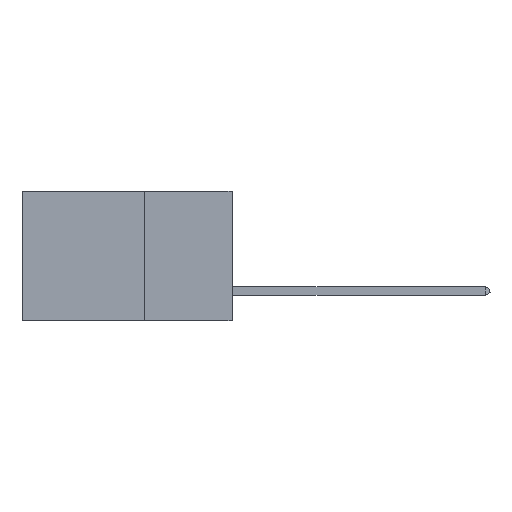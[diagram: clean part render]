
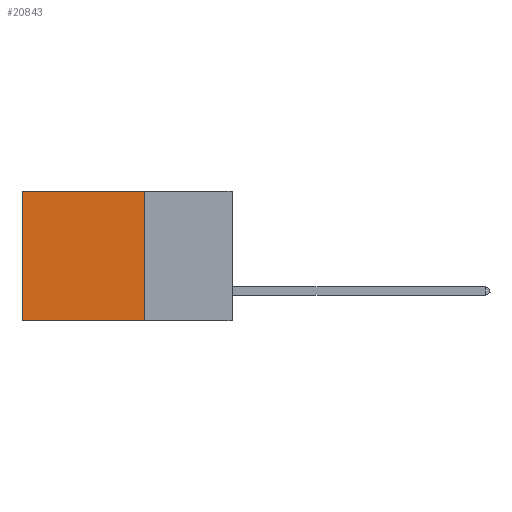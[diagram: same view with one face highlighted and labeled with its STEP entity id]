
A CAD part, left-side view. The second image highlights one B-rep face of the part: STEP entity #20843.
In plain terms, the highlighted planar face has unit normal (-1, 0, 0).
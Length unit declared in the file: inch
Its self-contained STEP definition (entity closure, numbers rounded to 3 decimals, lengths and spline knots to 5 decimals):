
#1390 = LINE ( 'NONE', #25113, #13001 ) ;
#1434 = EDGE_CURVE ( 'NONE', #14051, #10631, #1390, .T. ) ;
#2097 = DIRECTION ( 'NONE',  ( 0., 0., -1. ) ) ;
#3875 = LINE ( 'NONE', #4711, #16712 ) ;
#4231 = DIRECTION ( 'NONE',  ( 0., 1., 0. ) ) ;
#4318 = CARTESIAN_POINT ( 'NONE',  ( 0.2875, 0.25, -0.37 ) ) ;
#4711 = CARTESIAN_POINT ( 'NONE',  ( 0.2875, 0.25, 0. ) ) ;
#4756 = CARTESIAN_POINT ( 'NONE',  ( 0.2875, 0.6, 0. ) ) ;
#4985 = LINE ( 'NONE', #17967, #7149 ) ;
#5354 = LINE ( 'NONE', #4318, #6259 ) ;
#5360 = CARTESIAN_POINT ( 'NONE',  ( 0.2875, 0.6, -0.37 ) ) ;
#5842 = FACE_OUTER_BOUND ( 'NONE', #7116, .T. ) ;
#6259 = VECTOR ( 'NONE', #4231, 39.37008 ) ;
#7116 = EDGE_LOOP ( 'NONE', ( #17181, #24095, #25211, #17843 ) ) ;
#7149 = VECTOR ( 'NONE', #22436, 39.37008 ) ;
#8126 = DIRECTION ( 'NONE',  ( 1., 0., 0. ) ) ;
#10112 = EDGE_CURVE ( 'NONE', #25941, #14051, #3875, .T. ) ;
#10631 = VERTEX_POINT ( 'NONE', #5360 ) ;
#11457 = CARTESIAN_POINT ( 'NONE',  ( 0.2875, 0.25, -0.37 ) ) ;
#13001 = VECTOR ( 'NONE', #19041, 39.37008 ) ;
#14051 = VERTEX_POINT ( 'NONE', #4756 ) ;
#14631 = EDGE_CURVE ( 'NONE', #25941, #18382, #4985, .T. ) ;
#16712 = VECTOR ( 'NONE', #18845, 39.37008 ) ;
#17181 = ORIENTED_EDGE ( 'NONE', *, *, #1434, .T. ) ;
#17843 = ORIENTED_EDGE ( 'NONE', *, *, #10112, .T. ) ;
#17967 = CARTESIAN_POINT ( 'NONE',  ( 0.2875, 0.25, 0. ) ) ;
#18382 = VERTEX_POINT ( 'NONE', #11457 ) ;
#18692 = EDGE_CURVE ( 'NONE', #18382, #10631, #5354, .T. ) ;
#18845 = DIRECTION ( 'NONE',  ( 0., 1., 0. ) ) ;
#18889 = CARTESIAN_POINT ( 'NONE',  ( 0.2875, 0.25, 0. ) ) ;
#19041 = DIRECTION ( 'NONE',  ( 0., 0., -1. ) ) ;
#19965 = PLANE ( 'NONE',  #23425 ) ;
#20145 = CARTESIAN_POINT ( 'NONE',  ( 0.2875, 0.25, 0. ) ) ;
#20843 = ADVANCED_FACE ( 'NONE', ( #5842 ), #19965, .F. ) ;
#22436 = DIRECTION ( 'NONE',  ( 0., 0., -1. ) ) ;
#23425 = AXIS2_PLACEMENT_3D ( 'NONE', #20145, #8126, #2097 ) ;
#24095 = ORIENTED_EDGE ( 'NONE', *, *, #18692, .F. ) ;
#25113 = CARTESIAN_POINT ( 'NONE',  ( 0.2875, 0.6, 0. ) ) ;
#25211 = ORIENTED_EDGE ( 'NONE', *, *, #14631, .F. ) ;
#25941 = VERTEX_POINT ( 'NONE', #18889 ) ;
